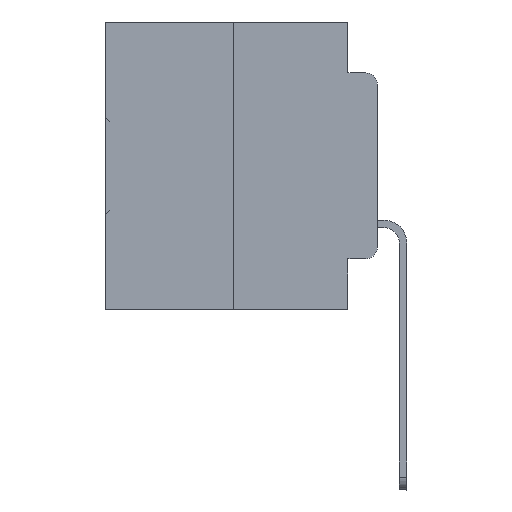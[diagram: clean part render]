
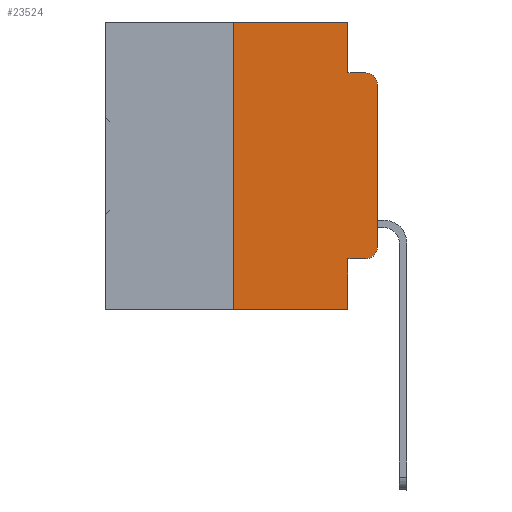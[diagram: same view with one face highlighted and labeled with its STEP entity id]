
A CAD part, left-side view. The second image highlights one B-rep face of the part: STEP entity #23524.
In plain terms, the highlighted planar face has unit normal (-1, 0, 0).
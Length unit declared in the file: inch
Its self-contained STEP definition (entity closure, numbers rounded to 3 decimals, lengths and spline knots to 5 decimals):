
#108 = ORIENTED_EDGE ( 'NONE', *, *, #4663, .T. ) ;
#522 = DIRECTION ( 'NONE',  ( 0., -1., 0. ) ) ;
#691 = CARTESIAN_POINT ( 'NONE',  ( 0., 0.02, -0.4115 ) ) ;
#1700 = DIRECTION ( 'NONE',  ( -1., 0., 0. ) ) ;
#2625 = CARTESIAN_POINT ( 'NONE',  ( 0., 0.051, 0. ) ) ;
#4020 = CARTESIAN_POINT ( 'NONE',  ( 0., 0.25, 0. ) ) ;
#4484 = DIRECTION ( 'NONE',  ( 0., -1., 0. ) ) ;
#4663 = EDGE_CURVE ( 'NONE', #15641, #6483, #15856, .T. ) ;
#4758 = DIRECTION ( 'NONE',  ( 0., -1., 0. ) ) ;
#5010 = VERTEX_POINT ( 'NONE', #18548 ) ;
#5609 = VECTOR ( 'NONE', #32583, 39.37008 ) ;
#5894 = CARTESIAN_POINT ( 'NONE',  ( 0., 0.051, -0.4115 ) ) ;
#6352 = ORIENTED_EDGE ( 'NONE', *, *, #16543, .T. ) ;
#6483 = VERTEX_POINT ( 'NONE', #691 ) ;
#6487 = DIRECTION ( 'NONE',  ( 0., 0., -1. ) ) ;
#6577 = ORIENTED_EDGE ( 'NONE', *, *, #12161, .F. ) ;
#7458 = VERTEX_POINT ( 'NONE', #33908 ) ;
#7558 = ORIENTED_EDGE ( 'NONE', *, *, #12819, .T. ) ;
#7713 = FACE_OUTER_BOUND ( 'NONE', #10001, .T. ) ;
#8513 = CARTESIAN_POINT ( 'NONE',  ( 0., 0.473, 0. ) ) ;
#8850 = EDGE_CURVE ( 'NONE', #21397, #25175, #20963, .T. ) ;
#9055 = CIRCLE ( 'NONE', #14093, 0.02 ) ;
#10001 = EDGE_LOOP ( 'NONE', ( #13665, #6352, #12825, #6577, #19558, #13126, #7558, #18188, #108, #10601 ) ) ;
#10268 = DIRECTION ( 'NONE',  ( 0., 0., -1. ) ) ;
#10469 = CARTESIAN_POINT ( 'NONE',  ( 0., 0.051, 0. ) ) ;
#10601 = ORIENTED_EDGE ( 'NONE', *, *, #33078, .T. ) ;
#11017 = CARTESIAN_POINT ( 'NONE',  ( 0., 0.051, -0.4115 ) ) ;
#11377 = VERTEX_POINT ( 'NONE', #20848 ) ;
#12161 = EDGE_CURVE ( 'NONE', #11377, #7458, #34262, .T. ) ;
#12819 = EDGE_CURVE ( 'NONE', #21397, #24780, #14647, .T. ) ;
#12825 = ORIENTED_EDGE ( 'NONE', *, *, #19315, .F. ) ;
#13084 = EDGE_CURVE ( 'NONE', #25175, #11377, #13749, .T. ) ;
#13126 = ORIENTED_EDGE ( 'NONE', *, *, #8850, .F. ) ;
#13665 = ORIENTED_EDGE ( 'NONE', *, *, #31771, .T. ) ;
#13691 = CIRCLE ( 'NONE', #24202, 0.02 ) ;
#13749 = LINE ( 'NONE', #8513, #13968 ) ;
#13968 = VECTOR ( 'NONE', #522, 39.37008 ) ;
#14093 = AXIS2_PLACEMENT_3D ( 'NONE', #27857, #22821, #6487 ) ;
#14383 = AXIS2_PLACEMENT_3D ( 'NONE', #31366, #18319, #15543 ) ;
#14647 = LINE ( 'NONE', #27169, #5609 ) ;
#15277 = VECTOR ( 'NONE', #21165, 39.37008 ) ;
#15543 = DIRECTION ( 'NONE',  ( 0., 0., -1. ) ) ;
#15641 = VERTEX_POINT ( 'NONE', #11017 ) ;
#15743 = CARTESIAN_POINT ( 'NONE',  ( 0., 0.25, 0. ) ) ;
#15856 = LINE ( 'NONE', #5894, #17347 ) ;
#16047 = CARTESIAN_POINT ( 'NONE',  ( 0., 0.051, -0.0885 ) ) ;
#16543 = EDGE_CURVE ( 'NONE', #23338, #29657, #9055, .T. ) ;
#16883 = CARTESIAN_POINT ( 'NONE',  ( 0., 0.051, -0.5 ) ) ;
#17002 = VECTOR ( 'NONE', #4484, 39.37008 ) ;
#17134 = EDGE_CURVE ( 'NONE', #15641, #24780, #33895, .T. ) ;
#17347 = VECTOR ( 'NONE', #4758, 39.37008 ) ;
#18188 = ORIENTED_EDGE ( 'NONE', *, *, #17134, .F. ) ;
#18319 = DIRECTION ( 'NONE',  ( 1., 0., 0. ) ) ;
#18372 = VECTOR ( 'NONE', #30995, 39.37008 ) ;
#18548 = CARTESIAN_POINT ( 'NONE',  ( 0., 0., -0.3915 ) ) ;
#18560 = VECTOR ( 'NONE', #10268, 39.37008 ) ;
#19315 = EDGE_CURVE ( 'NONE', #7458, #29657, #32206, .T. ) ;
#19558 = ORIENTED_EDGE ( 'NONE', *, *, #13084, .F. ) ;
#20284 = CARTESIAN_POINT ( 'NONE',  ( 0., 0.02, -0.3915 ) ) ;
#20757 = PLANE ( 'NONE',  #14383 ) ;
#20848 = CARTESIAN_POINT ( 'NONE',  ( 0., 0.051, 0. ) ) ;
#20963 = LINE ( 'NONE', #15743, #27303 ) ;
#21165 = DIRECTION ( 'NONE',  ( 0., 0., 1. ) ) ;
#21397 = VERTEX_POINT ( 'NONE', #29850 ) ;
#22821 = DIRECTION ( 'NONE',  ( -1., 0., 0. ) ) ;
#23338 = VERTEX_POINT ( 'NONE', #32592 ) ;
#23524 = ADVANCED_FACE ( 'NONE', ( #7713 ), #20757, .F. ) ;
#24202 = AXIS2_PLACEMENT_3D ( 'NONE', #20284, #1700, #30555 ) ;
#24780 = VERTEX_POINT ( 'NONE', #16883 ) ;
#25175 = VERTEX_POINT ( 'NONE', #4020 ) ;
#25988 = DIRECTION ( 'NONE',  ( 0., 0., 1. ) ) ;
#26777 = CARTESIAN_POINT ( 'NONE',  ( 0., 0.02, -0.0885 ) ) ;
#27169 = CARTESIAN_POINT ( 'NONE',  ( 0., 0.473, -0.5 ) ) ;
#27303 = VECTOR ( 'NONE', #25988, 39.37008 ) ;
#27857 = CARTESIAN_POINT ( 'NONE',  ( 0., 0.02, -0.1085 ) ) ;
#29657 = VERTEX_POINT ( 'NONE', #26777 ) ;
#29850 = CARTESIAN_POINT ( 'NONE',  ( 0., 0.25, -0.5 ) ) ;
#30555 = DIRECTION ( 'NONE',  ( 0., 0., -1. ) ) ;
#30995 = DIRECTION ( 'NONE',  ( 0., 0., -1. ) ) ;
#31366 = CARTESIAN_POINT ( 'NONE',  ( 0., 0.473, 0. ) ) ;
#31609 = LINE ( 'NONE', #31949, #15277 ) ;
#31771 = EDGE_CURVE ( 'NONE', #5010, #23338, #31609, .T. ) ;
#31949 = CARTESIAN_POINT ( 'NONE',  ( 0., 0., 0. ) ) ;
#32206 = LINE ( 'NONE', #16047, #17002 ) ;
#32583 = DIRECTION ( 'NONE',  ( 0., -1., 0. ) ) ;
#32592 = CARTESIAN_POINT ( 'NONE',  ( 0., 0., -0.1085 ) ) ;
#33078 = EDGE_CURVE ( 'NONE', #6483, #5010, #13691, .T. ) ;
#33895 = LINE ( 'NONE', #2625, #18560 ) ;
#33908 = CARTESIAN_POINT ( 'NONE',  ( 0., 0.051, -0.0885 ) ) ;
#34262 = LINE ( 'NONE', #10469, #18372 ) ;
